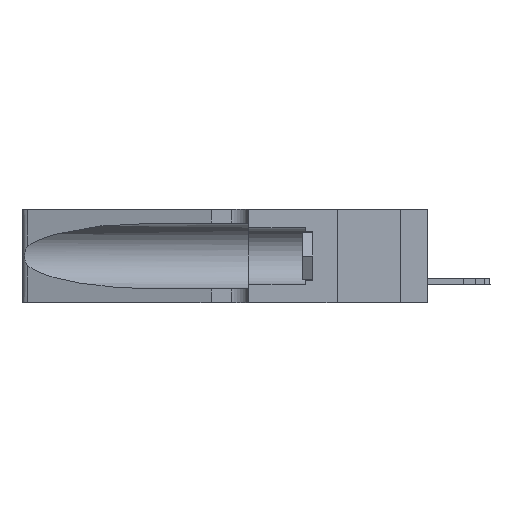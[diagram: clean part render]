
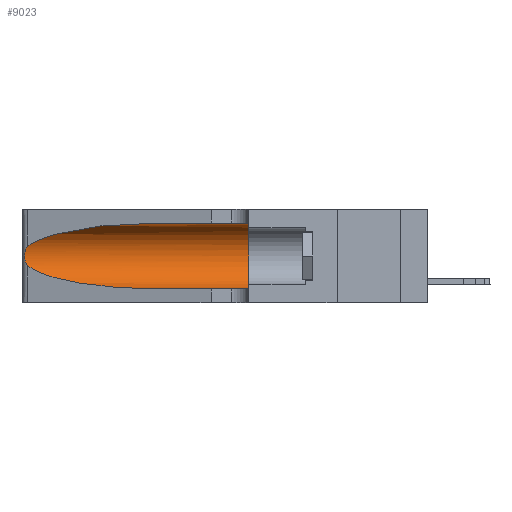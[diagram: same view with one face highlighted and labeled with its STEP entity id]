
A CAD part, left-side view. The second image highlights one B-rep face of the part: STEP entity #9023.
In plain terms, the highlighted cylindrical face has radius 3.308 mm (diameter 6.617 mm), a partial arc.
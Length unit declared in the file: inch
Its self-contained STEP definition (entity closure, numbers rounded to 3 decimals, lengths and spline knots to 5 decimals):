
#1222 = CARTESIAN_POINT ( 'NONE',  ( 0.25639, 1.23184, 0.21858 ) ) ;
#1556 = CARTESIAN_POINT ( 'NONE',  ( 0.26075, 1.23896, 0.19203 ) ) ;
#2947 = DIRECTION ( 'NONE',  ( 0., -1., 0. ) ) ;
#4386 = CARTESIAN_POINT ( 'NONE',  ( 0.26018, 1.23835, 0.19895 ) ) ;
#4570 = ORIENTED_EDGE ( 'NONE', *, *, #22727, .F. ) ;
#4692 = CIRCLE ( 'NONE', #10916, 0.13025 ) ;
#4779 = CARTESIAN_POINT ( 'NONE',  ( 0.25487, 1.22718, 0.22369 ) ) ;
#5607 = AXIS2_PLACEMENT_3D ( 'NONE', #15954, #2947, #29333 ) ;
#6438 = VERTEX_POINT ( 'NONE', #17362 ) ;
#6487 = CARTESIAN_POINT ( 'NONE',  ( 0.1305, 0.35, 0.05475 ) ) ;
#6584 = DIRECTION ( 'NONE',  ( 0., 0., 1. ) ) ;
#6893 = CARTESIAN_POINT ( 'NONE',  ( 0.26075, 1.23896, 0.178 ) ) ;
#8287 = VECTOR ( 'NONE', #21966, 39.37008 ) ;
#9023 = ADVANCED_FACE ( 'NONE', ( #9203 ), #22683, .F. ) ;
#9203 = FACE_OUTER_BOUND ( 'NONE', #23169, .T. ) ;
#9657 = VERTEX_POINT ( 'NONE', #33499 ) ;
#10536 = EDGE_CURVE ( 'NONE', #9657, #6438, #26963, .T. ) ;
#10916 = AXIS2_PLACEMENT_3D ( 'NONE', #22198, #14452, #6584 ) ;
#10942 = ORIENTED_EDGE ( 'NONE', *, *, #11570, .T. ) ;
#10960 = CARTESIAN_POINT ( 'NONE',  ( 0.18966, 0.96281, 0.05475 ) ) ;
#11570 = EDGE_CURVE ( 'NONE', #13314, #9657, #21893, .T. ) ;
#11621 = VECTOR ( 'NONE', #30112, 39.37008 ) ;
#11948 = CARTESIAN_POINT ( 'NONE',  ( 0.25787, 1.23484, 0.2124 ) ) ;
#12180 = VERTEX_POINT ( 'NONE', #32672 ) ;
#12270 = CARTESIAN_POINT ( 'NONE',  ( 0.25487, 1.22718, 0.14631 ) ) ;
#12408 = VERTEX_POINT ( 'NONE', #21832 ) ;
#12435 = CARTESIAN_POINT ( 'NONE',  ( 0.1305, 0.72297, 0.31525 ) ) ;
#13314 = VERTEX_POINT ( 'NONE', #31975 ) ;
#13440 = CARTESIAN_POINT ( 'NONE',  ( 0.25487, 1.22718, 0.14631 ) ) ;
#13711 =( BOUNDED_CURVE ( )  B_SPLINE_CURVE ( 3, ( #12435, #15264, #20155, #4779 ),
 .UNSPECIFIED., .F., .T. ) 
 B_SPLINE_CURVE_WITH_KNOTS ( ( 4, 4 ),
 ( 1.5708, 2.84003 ),
 .UNSPECIFIED. ) 
 CURVE ( )  GEOMETRIC_REPRESENTATION_ITEM ( )  RATIONAL_B_SPLINE_CURVE ( ( 1., 0.87, 0.87, 1. ) ) 
 REPRESENTATION_ITEM ( '' )  );
#14452 = DIRECTION ( 'NONE',  ( 0., 1., 0. ) ) ;
#15264 = CARTESIAN_POINT ( 'NONE',  ( 0.18966, 0.96281, 0.31525 ) ) ;
#15758 = EDGE_CURVE ( 'NONE', #12408, #12180, #31691, .T. ) ;
#15954 = CARTESIAN_POINT ( 'NONE',  ( 0.1305, 1.61858, 0.185 ) ) ;
#16160 = EDGE_CURVE ( 'NONE', #6438, #21998, #23444, .T. ) ;
#16811 = CARTESIAN_POINT ( 'NONE',  ( 0.25487, 1.22718, 0.22369 ) ) ;
#17223 = ORIENTED_EDGE ( 'NONE', *, *, #10536, .T. ) ;
#17362 = CARTESIAN_POINT ( 'NONE',  ( 0.1305, 0.72297, 0.05475 ) ) ;
#17502 = CARTESIAN_POINT ( 'NONE',  ( 0.26017, 1.23833, 0.17102 ) ) ;
#18239 = CARTESIAN_POINT ( 'NONE',  ( 0.1305, 0.72297, 0.05475 ) ) ;
#19346 = CARTESIAN_POINT ( 'NONE',  ( 0.1305, 1.61858, 0.05475 ) ) ;
#20155 = CARTESIAN_POINT ( 'NONE',  ( 0.2373, 1.15595, 0.28018 ) ) ;
#21832 = CARTESIAN_POINT ( 'NONE',  ( 0.1305, 0.72297, 0.31525 ) ) ;
#21835 = CARTESIAN_POINT ( 'NONE',  ( 0.25555, 1.22994, 0.2215 ) ) ;
#21893 = B_SPLINE_CURVE_WITH_KNOTS ( 'NONE', 3,
 ( #16811, #21835, #1222, #11948, #22860, #4386, #1556, #6893, #17502, #30234, #24939, #32859, #27912, #12270 ),
 .UNSPECIFIED., .F., .F.,
 ( 4, 2, 2, 2, 2, 2, 4 ),
 ( 0., 0.00027, 0.00053, 0.00107, 0.0016, 0.00187, 0.00214 ),
 .UNSPECIFIED. ) ;
#21966 = DIRECTION ( 'NONE',  ( 0., -1., 0. ) ) ;
#21998 = VERTEX_POINT ( 'NONE', #6487 ) ;
#22198 = CARTESIAN_POINT ( 'NONE',  ( 0.1305, 0.35, 0.185 ) ) ;
#22683 = CYLINDRICAL_SURFACE ( 'NONE', #5607, 0.13025 ) ;
#22727 = EDGE_CURVE ( 'NONE', #12180, #21998, #4692, .T. ) ;
#22756 = ORIENTED_EDGE ( 'NONE', *, *, #15758, .F. ) ;
#22860 = CARTESIAN_POINT ( 'NONE',  ( 0.25854, 1.2359, 0.20912 ) ) ;
#23169 = EDGE_LOOP ( 'NONE', ( #25350, #10942, #17223, #24486, #4570, #22756 ) ) ;
#23444 = LINE ( 'NONE', #19346, #8287 ) ;
#24486 = ORIENTED_EDGE ( 'NONE', *, *, #16160, .T. ) ;
#24939 = CARTESIAN_POINT ( 'NONE',  ( 0.25789, 1.23486, 0.15765 ) ) ;
#25350 = ORIENTED_EDGE ( 'NONE', *, *, #25894, .T. ) ;
#25894 = EDGE_CURVE ( 'NONE', #12408, #13314, #13711, .T. ) ;
#26963 =( BOUNDED_CURVE ( )  B_SPLINE_CURVE ( 3, ( #13440, #31784, #10960, #18239 ),
 .UNSPECIFIED., .F., .F. ) 
 B_SPLINE_CURVE_WITH_KNOTS ( ( 4, 4 ),
 ( 3.44316, 4.71239 ),
 .UNSPECIFIED. ) 
 CURVE ( )  GEOMETRIC_REPRESENTATION_ITEM ( )  RATIONAL_B_SPLINE_CURVE ( ( 1., 0.87, 0.87, 1. ) ) 
 REPRESENTATION_ITEM ( '' )  );
#27912 = CARTESIAN_POINT ( 'NONE',  ( 0.25555, 1.22993, 0.14849 ) ) ;
#29333 = DIRECTION ( 'NONE',  ( 0., 0., -1. ) ) ;
#30112 = DIRECTION ( 'NONE',  ( 0., -1., 0. ) ) ;
#30234 = CARTESIAN_POINT ( 'NONE',  ( 0.25856, 1.23593, 0.16098 ) ) ;
#30443 = CARTESIAN_POINT ( 'NONE',  ( 0.1305, 1.61858, 0.31525 ) ) ;
#31691 = LINE ( 'NONE', #30443, #11621 ) ;
#31784 = CARTESIAN_POINT ( 'NONE',  ( 0.2373, 1.15595, 0.08982 ) ) ;
#31975 = CARTESIAN_POINT ( 'NONE',  ( 0.25487, 1.22718, 0.22369 ) ) ;
#32672 = CARTESIAN_POINT ( 'NONE',  ( 0.1305, 0.35, 0.31525 ) ) ;
#32859 = CARTESIAN_POINT ( 'NONE',  ( 0.25639, 1.23186, 0.15144 ) ) ;
#33499 = CARTESIAN_POINT ( 'NONE',  ( 0.25487, 1.22718, 0.14631 ) ) ;
